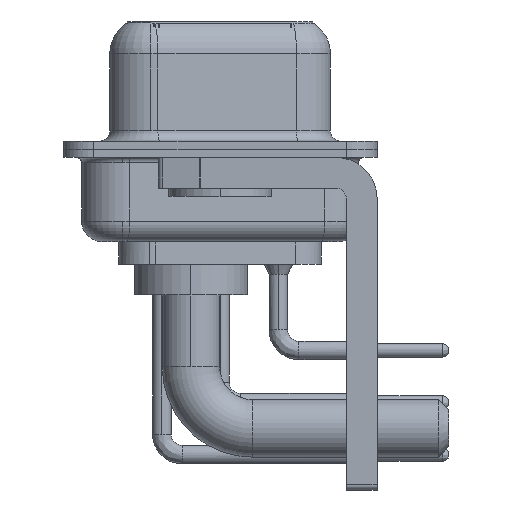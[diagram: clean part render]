
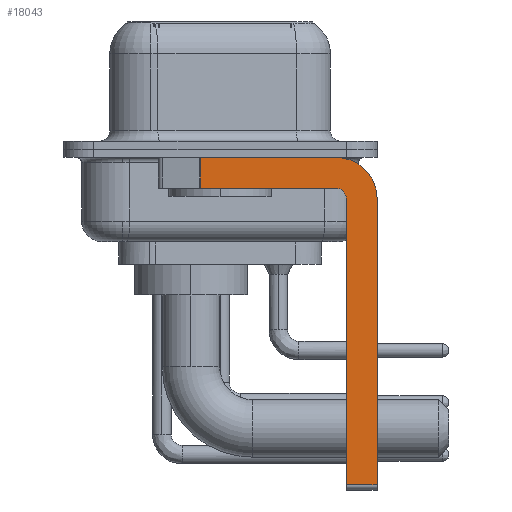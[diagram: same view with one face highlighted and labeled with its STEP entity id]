
A CAD part, left-side view. The second image highlights one B-rep face of the part: STEP entity #18043.
In plain terms, the highlighted planar face has unit normal (-1, 0, 0).
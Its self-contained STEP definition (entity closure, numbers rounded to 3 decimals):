
#164 = CARTESIAN_POINT ( 'NONE',  ( -2.9, -6.15, -16.6 ) ) ;
#890 = ORIENTED_EDGE ( 'NONE', *, *, #15870, .F. ) ;
#1561 = CIRCLE ( 'NONE', #8879, 2. ) ;
#3108 = VERTEX_POINT ( 'NONE', #21436 ) ;
#3205 = DIRECTION ( 'NONE',  ( 0., 0., -1. ) ) ;
#3495 = EDGE_CURVE ( 'NONE', #28314, #3108, #28665, .T. ) ;
#3698 = ORIENTED_EDGE ( 'NONE', *, *, #15405, .T. ) ;
#3774 = CARTESIAN_POINT ( 'NONE',  ( -2.9, 0.978, -0.4 ) ) ;
#4023 = AXIS2_PLACEMENT_3D ( 'NONE', #22357, #29205, #8354 ) ;
#5390 = VECTOR ( 'NONE', #14732, 1000. ) ;
#5416 = CARTESIAN_POINT ( 'NONE',  ( -2.9, 0.978, -1.9 ) ) ;
#5431 = VERTEX_POINT ( 'NONE', #6372 ) ;
#5626 = CARTESIAN_POINT ( 'NONE',  ( -2.9, 3., -0.4 ) ) ;
#5776 = DIRECTION ( 'NONE',  ( -1., 0., 0. ) ) ;
#6236 = DIRECTION ( 'NONE',  ( 0., 1., 0. ) ) ;
#6372 = CARTESIAN_POINT ( 'NONE',  ( -2.9, -5.65, -1.9 ) ) ;
#6553 = EDGE_CURVE ( 'NONE', #29654, #27188, #28356, .T. ) ;
#6615 = CARTESIAN_POINT ( 'NONE',  ( -2.9, -6.15, -2.4 ) ) ;
#6660 = EDGE_CURVE ( 'NONE', #10489, #29194, #28654, .T. ) ;
#7261 = EDGE_CURVE ( 'NONE', #29194, #28314, #1561, .T. ) ;
#7785 = DIRECTION ( 'NONE',  ( 0., -1., 0. ) ) ;
#8103 = ORIENTED_EDGE ( 'NONE', *, *, #6660, .F. ) ;
#8354 = DIRECTION ( 'NONE',  ( 0., 0., -1. ) ) ;
#8522 = AXIS2_PLACEMENT_3D ( 'NONE', #26813, #5776, #17842 ) ;
#8879 = AXIS2_PLACEMENT_3D ( 'NONE', #29508, #20529, #29664 ) ;
#10178 = LINE ( 'NONE', #12318, #11061 ) ;
#10489 = VERTEX_POINT ( 'NONE', #3774 ) ;
#10632 = FACE_OUTER_BOUND ( 'NONE', #13953, .T. ) ;
#11061 = VECTOR ( 'NONE', #24335, 1000. ) ;
#12318 = CARTESIAN_POINT ( 'NONE',  ( -2.9, -5.65, -16.35 ) ) ;
#12445 = ORIENTED_EDGE ( 'NONE', *, *, #26453, .T. ) ;
#12502 = CARTESIAN_POINT ( 'NONE',  ( -2.9, -7.65, -2.4 ) ) ;
#12908 = ORIENTED_EDGE ( 'NONE', *, *, #3495, .F. ) ;
#13370 = CARTESIAN_POINT ( 'NONE',  ( -2.9, -5.65, -0.4 ) ) ;
#13703 = VECTOR ( 'NONE', #7785, 1000. ) ;
#13953 = EDGE_LOOP ( 'NONE', ( #8103, #3698, #890, #23971, #24017, #12445, #12908, #19327 ) ) ;
#14732 = DIRECTION ( 'NONE',  ( 0., 0., -1. ) ) ;
#15405 = EDGE_CURVE ( 'NONE', #10489, #28085, #26287, .T. ) ;
#15870 = EDGE_CURVE ( 'NONE', #5431, #28085, #27436, .T. ) ;
#17310 = CARTESIAN_POINT ( 'NONE',  ( -2.9, 0.978, -1.9 ) ) ;
#17842 = DIRECTION ( 'NONE',  ( 0., 0., 1. ) ) ;
#18043 = ADVANCED_FACE ( 'NONE', ( #10632 ), #22512, .F. ) ;
#18773 = DIRECTION ( 'NONE',  ( 0., 0., 1. ) ) ;
#19327 = ORIENTED_EDGE ( 'NONE', *, *, #7261, .F. ) ;
#20529 = DIRECTION ( 'NONE',  ( 1., 0., 0. ) ) ;
#20991 = VECTOR ( 'NONE', #18773, 1000. ) ;
#21436 = CARTESIAN_POINT ( 'NONE',  ( -2.9, -7.65, -16.35 ) ) ;
#22357 = CARTESIAN_POINT ( 'NONE',  ( -2.9, -5.65, -2.4 ) ) ;
#22364 = EDGE_CURVE ( 'NONE', #27188, #5431, #27970, .T. ) ;
#22512 = PLANE ( 'NONE',  #4023 ) ;
#22765 = CARTESIAN_POINT ( 'NONE',  ( -2.9, -7.65, -2.4 ) ) ;
#23971 = ORIENTED_EDGE ( 'NONE', *, *, #22364, .F. ) ;
#24017 = ORIENTED_EDGE ( 'NONE', *, *, #6553, .F. ) ;
#24335 = DIRECTION ( 'NONE',  ( 0., -1., 0. ) ) ;
#24834 = CARTESIAN_POINT ( 'NONE',  ( -2.9, -5.65, -1.9 ) ) ;
#26287 = LINE ( 'NONE', #5416, #5390 ) ;
#26453 = EDGE_CURVE ( 'NONE', #29654, #3108, #10178, .T. ) ;
#26813 = CARTESIAN_POINT ( 'NONE',  ( -2.9, -5.65, -2.4 ) ) ;
#27056 = VECTOR ( 'NONE', #3205, 1000. ) ;
#27188 = VERTEX_POINT ( 'NONE', #6615 ) ;
#27436 = LINE ( 'NONE', #24834, #27824 ) ;
#27824 = VECTOR ( 'NONE', #6236, 1000. ) ;
#27970 = CIRCLE ( 'NONE', #8522, 0.5 ) ;
#28085 = VERTEX_POINT ( 'NONE', #17310 ) ;
#28314 = VERTEX_POINT ( 'NONE', #22765 ) ;
#28356 = LINE ( 'NONE', #164, #20991 ) ;
#28654 = LINE ( 'NONE', #5626, #13703 ) ;
#28665 = LINE ( 'NONE', #12502, #27056 ) ;
#29194 = VERTEX_POINT ( 'NONE', #13370 ) ;
#29205 = DIRECTION ( 'NONE',  ( 1., 0., 0. ) ) ;
#29508 = CARTESIAN_POINT ( 'NONE',  ( -2.9, -5.65, -2.4 ) ) ;
#29654 = VERTEX_POINT ( 'NONE', #30071 ) ;
#29664 = DIRECTION ( 'NONE',  ( 0., 0., -1. ) ) ;
#30071 = CARTESIAN_POINT ( 'NONE',  ( -2.9, -6.15, -16.35 ) ) ;
